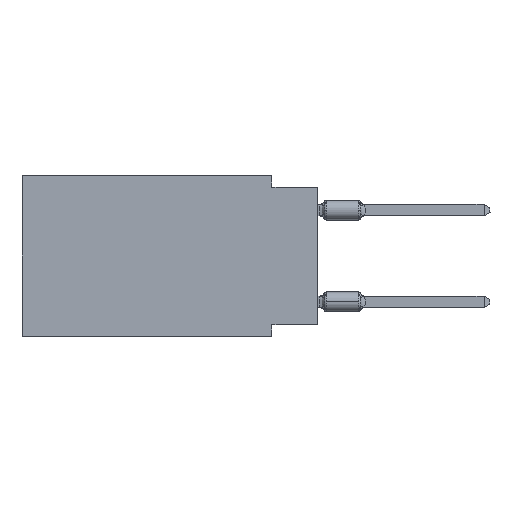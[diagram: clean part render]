
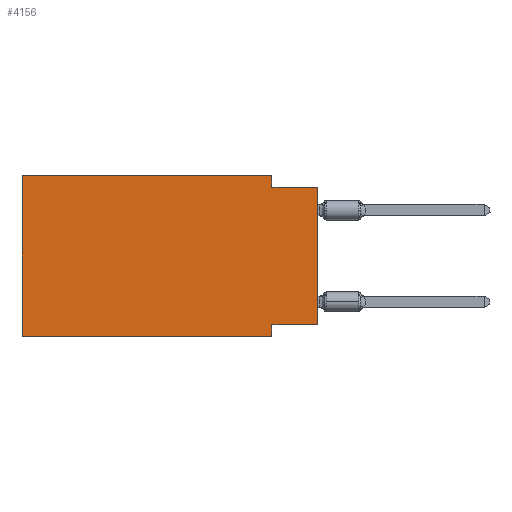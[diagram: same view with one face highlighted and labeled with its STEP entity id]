
A CAD part, left-side view. The second image highlights one B-rep face of the part: STEP entity #4156.
In plain terms, the highlighted planar face has unit normal (-1, 0, 0).
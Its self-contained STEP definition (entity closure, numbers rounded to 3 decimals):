
#464 = DIRECTION ( 'NONE',  ( 0., -1., 0. ) ) ;
#1065 = CARTESIAN_POINT ( 'NONE',  ( 0., 0., -8.255 ) ) ;
#2272 = VERTEX_POINT ( 'NONE', #48462 ) ;
#3151 = EDGE_CURVE ( 'NONE', #17980, #39401, #25975, .T. ) ;
#3318 = CARTESIAN_POINT ( 'NONE',  ( 0., 2.54, 0. ) ) ;
#3697 = DIRECTION ( 'NONE',  ( 0., -1., 0. ) ) ;
#4156 = ADVANCED_FACE ( 'NONE', ( #40968 ), #14345, .F. ) ;
#4237 = EDGE_CURVE ( 'NONE', #11025, #18867, #35489, .T. ) ;
#5220 = LINE ( 'NONE', #20815, #39453 ) ;
#5661 = DIRECTION ( 'NONE',  ( 0., 1., 0. ) ) ;
#6782 = VECTOR ( 'NONE', #11224, 1000. ) ;
#6792 = VECTOR ( 'NONE', #5661, 1000. ) ;
#7492 = ORIENTED_EDGE ( 'NONE', *, *, #26742, .T. ) ;
#8741 = CARTESIAN_POINT ( 'NONE',  ( 0., 0., -0.635 ) ) ;
#9053 = CARTESIAN_POINT ( 'NONE',  ( 0., 2.54, -8.89 ) ) ;
#9936 = CARTESIAN_POINT ( 'NONE',  ( 0., 16.383, 0. ) ) ;
#10344 = ORIENTED_EDGE ( 'NONE', *, *, #33360, .F. ) ;
#10499 = CARTESIAN_POINT ( 'NONE',  ( 0., 16.383, 0. ) ) ;
#11025 = VERTEX_POINT ( 'NONE', #14814 ) ;
#11061 = ORIENTED_EDGE ( 'NONE', *, *, #38589, .F. ) ;
#11224 = DIRECTION ( 'NONE',  ( 0., 0., -1. ) ) ;
#12700 = LINE ( 'NONE', #28325, #26673 ) ;
#12829 = LINE ( 'NONE', #8741, #40394 ) ;
#13170 = EDGE_LOOP ( 'NONE', ( #7492, #13233, #19863, #43049, #11061, #14557, #36285, #10344 ) ) ;
#13233 = ORIENTED_EDGE ( 'NONE', *, *, #19239, .F. ) ;
#14211 = CARTESIAN_POINT ( 'NONE',  ( 0., 0., -0.635 ) ) ;
#14323 = LINE ( 'NONE', #3318, #6782 ) ;
#14345 = PLANE ( 'NONE',  #36860 ) ;
#14557 = ORIENTED_EDGE ( 'NONE', *, *, #4237, .T. ) ;
#14814 = CARTESIAN_POINT ( 'NONE',  ( 0., 16.383, -8.89 ) ) ;
#16612 = CARTESIAN_POINT ( 'NONE',  ( 0., 2.54, 0. ) ) ;
#17980 = VERTEX_POINT ( 'NONE', #9936 ) ;
#18867 = VERTEX_POINT ( 'NONE', #9053 ) ;
#19239 = EDGE_CURVE ( 'NONE', #2272, #34304, #12829, .T. ) ;
#19863 = ORIENTED_EDGE ( 'NONE', *, *, #26887, .F. ) ;
#20637 = DIRECTION ( 'NONE',  ( 0., 0., 1. ) ) ;
#20815 = CARTESIAN_POINT ( 'NONE',  ( 0., 0., 0. ) ) ;
#23992 = CARTESIAN_POINT ( 'NONE',  ( 0., 16.383, -8.89 ) ) ;
#25975 = LINE ( 'NONE', #34384, #40831 ) ;
#26673 = VECTOR ( 'NONE', #20637, 1000. ) ;
#26742 = EDGE_CURVE ( 'NONE', #27307, #34304, #5220, .T. ) ;
#26887 = EDGE_CURVE ( 'NONE', #39401, #2272, #14323, .T. ) ;
#27307 = VERTEX_POINT ( 'NONE', #37792 ) ;
#28325 = CARTESIAN_POINT ( 'NONE',  ( 0., 16.383, 0. ) ) ;
#33035 = VECTOR ( 'NONE', #48150, 1000. ) ;
#33046 = DIRECTION ( 'NONE',  ( 0., -1., 0. ) ) ;
#33360 = EDGE_CURVE ( 'NONE', #27307, #40385, #44810, .T. ) ;
#34304 = VERTEX_POINT ( 'NONE', #14211 ) ;
#34384 = CARTESIAN_POINT ( 'NONE',  ( 0., 16.383, 0. ) ) ;
#35489 = LINE ( 'NONE', #23992, #43403 ) ;
#36285 = ORIENTED_EDGE ( 'NONE', *, *, #44193, .F. ) ;
#36416 = DIRECTION ( 'NONE',  ( 0., 0., 1. ) ) ;
#36860 = AXIS2_PLACEMENT_3D ( 'NONE', #10499, #48440, #36883 ) ;
#36883 = DIRECTION ( 'NONE',  ( 0., 0., -1. ) ) ;
#37563 = CARTESIAN_POINT ( 'NONE',  ( 0., 2.54, -8.255 ) ) ;
#37792 = CARTESIAN_POINT ( 'NONE',  ( 0., 0., -8.255 ) ) ;
#38589 = EDGE_CURVE ( 'NONE', #11025, #17980, #12700, .T. ) ;
#39401 = VERTEX_POINT ( 'NONE', #16612 ) ;
#39453 = VECTOR ( 'NONE', #36416, 1000. ) ;
#40385 = VERTEX_POINT ( 'NONE', #37563 ) ;
#40394 = VECTOR ( 'NONE', #33046, 1000. ) ;
#40831 = VECTOR ( 'NONE', #3697, 1000. ) ;
#40968 = FACE_OUTER_BOUND ( 'NONE', #13170, .T. ) ;
#43049 = ORIENTED_EDGE ( 'NONE', *, *, #3151, .F. ) ;
#43403 = VECTOR ( 'NONE', #464, 1000. ) ;
#44035 = LINE ( 'NONE', #44805, #33035 ) ;
#44193 = EDGE_CURVE ( 'NONE', #40385, #18867, #44035, .T. ) ;
#44805 = CARTESIAN_POINT ( 'NONE',  ( 0., 2.54, -8.89 ) ) ;
#44810 = LINE ( 'NONE', #1065, #6792 ) ;
#48150 = DIRECTION ( 'NONE',  ( 0., 0., -1. ) ) ;
#48440 = DIRECTION ( 'NONE',  ( 1., 0., 0. ) ) ;
#48462 = CARTESIAN_POINT ( 'NONE',  ( 0., 2.54, -0.635 ) ) ;
